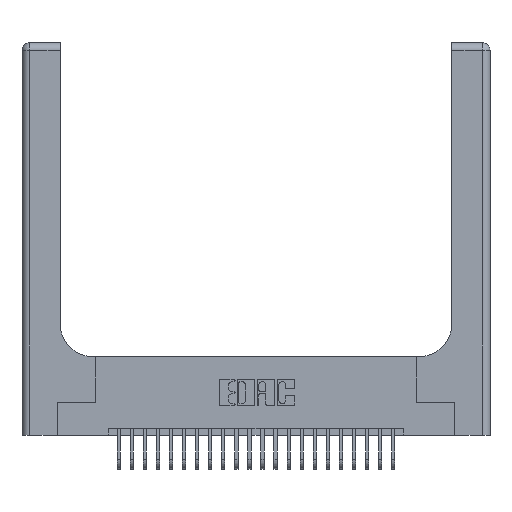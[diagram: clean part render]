
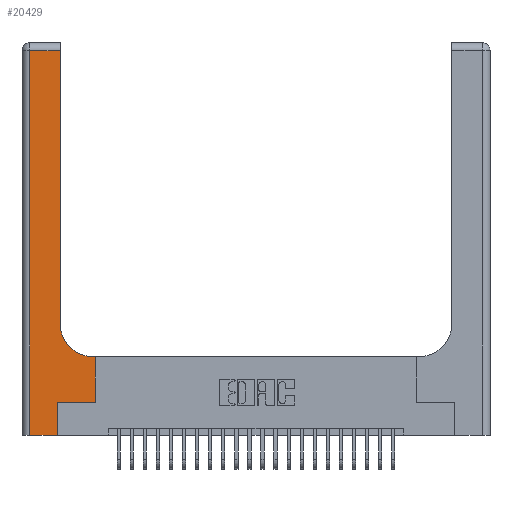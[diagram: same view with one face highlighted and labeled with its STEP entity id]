
A CAD part, top view. The second image highlights one B-rep face of the part: STEP entity #20429.
In plain terms, the highlighted planar face has unit normal (0, 0, 1).
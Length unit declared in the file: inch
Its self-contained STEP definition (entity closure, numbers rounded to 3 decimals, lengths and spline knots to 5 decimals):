
#348 = CARTESIAN_POINT ( 'NONE',  ( 0.2915, 3., 0.37 ) ) ;
#373 = VECTOR ( 'NONE', #18323, 39.37008 ) ;
#494 = ORIENTED_EDGE ( 'NONE', *, *, #7584, .T. ) ;
#872 = CARTESIAN_POINT ( 'NONE',  ( 0.2915, 0.6, 0.37 ) ) ;
#1083 = VECTOR ( 'NONE', #22048, 39.37008 ) ;
#1438 = DIRECTION ( 'NONE',  ( 0., -1., 0. ) ) ;
#1998 = VECTOR ( 'NONE', #5953, 39.37008 ) ;
#2379 = EDGE_CURVE ( 'NONE', #13437, #9790, #12954, .T. ) ;
#2691 = VERTEX_POINT ( 'NONE', #5757 ) ;
#2952 = VECTOR ( 'NONE', #17506, 39.37008 ) ;
#3462 = VECTOR ( 'NONE', #1438, 39.37008 ) ;
#3975 = DIRECTION ( 'NONE',  ( 1., 0., 0. ) ) ;
#4070 = CARTESIAN_POINT ( 'NONE',  ( 0.269, 0.25, 0.37 ) ) ;
#4483 = EDGE_CURVE ( 'NONE', #10352, #2691, #19727, .T. ) ;
#4904 = AXIS2_PLACEMENT_3D ( 'NONE', #17351, #9272, #21619 ) ;
#5395 = CARTESIAN_POINT ( 'NONE',  ( 0.269, 0., 0.37 ) ) ;
#5524 = FACE_OUTER_BOUND ( 'NONE', #23906, .T. ) ;
#5757 = CARTESIAN_POINT ( 'NONE',  ( 0.2915, 2.94, 0.37 ) ) ;
#5821 = DIRECTION ( 'NONE',  ( 1., 0., 0. ) ) ;
#5953 = DIRECTION ( 'NONE',  ( -1., 0., 0. ) ) ;
#6017 = LINE ( 'NONE', #18835, #8884 ) ;
#6260 = ORIENTED_EDGE ( 'NONE', *, *, #2379, .T. ) ;
#6697 = DIRECTION ( 'NONE',  ( 0., 1., 0. ) ) ;
#6886 = VERTEX_POINT ( 'NONE', #24408 ) ;
#7006 = CARTESIAN_POINT ( 'NONE',  ( 0.5585, 0.25, 0.37 ) ) ;
#7324 = CARTESIAN_POINT ( 'NONE',  ( 0.5585, 0.6, 0.37 ) ) ;
#7468 = VERTEX_POINT ( 'NONE', #17929 ) ;
#7551 = CARTESIAN_POINT ( 'NONE',  ( 0.5415, 0.6, 0.37 ) ) ;
#7584 = EDGE_CURVE ( 'NONE', #19217, #7468, #12005, .T. ) ;
#7746 = ORIENTED_EDGE ( 'NONE', *, *, #4483, .T. ) ;
#8631 = ORIENTED_EDGE ( 'NONE', *, *, #8891, .T. ) ;
#8880 = CARTESIAN_POINT ( 'NONE',  ( 0., 0., 0.37 ) ) ;
#8884 = VECTOR ( 'NONE', #6697, 39.37008 ) ;
#8891 = EDGE_CURVE ( 'NONE', #16024, #10560, #21038, .T. ) ;
#9272 = DIRECTION ( 'NONE',  ( 0., 0., -1. ) ) ;
#9406 = LINE ( 'NONE', #16996, #1998 ) ;
#9558 = LINE ( 'NONE', #24699, #3462 ) ;
#9790 = VERTEX_POINT ( 'NONE', #7551 ) ;
#9895 = ORIENTED_EDGE ( 'NONE', *, *, #23053, .T. ) ;
#10352 = VERTEX_POINT ( 'NONE', #20778 ) ;
#10560 = VERTEX_POINT ( 'NONE', #7006 ) ;
#10814 = EDGE_CURVE ( 'NONE', #6886, #19217, #9558, .T. ) ;
#10917 = VECTOR ( 'NONE', #14787, 39.37008 ) ;
#12005 = LINE ( 'NONE', #8880, #373 ) ;
#12451 = ORIENTED_EDGE ( 'NONE', *, *, #15175, .T. ) ;
#12764 = CIRCLE ( 'NONE', #25230, 0.25 ) ;
#12954 = LINE ( 'NONE', #872, #2952 ) ;
#13437 = VERTEX_POINT ( 'NONE', #7324 ) ;
#14045 = DIRECTION ( 'NONE',  ( 0., 0., -1. ) ) ;
#14787 = DIRECTION ( 'NONE',  ( 0., 1., 0. ) ) ;
#15175 = EDGE_CURVE ( 'NONE', #2691, #6886, #9406, .T. ) ;
#15218 = CARTESIAN_POINT ( 'NONE',  ( 0.269, 0.25, 0.37 ) ) ;
#16024 = VERTEX_POINT ( 'NONE', #15218 ) ;
#16996 = CARTESIAN_POINT ( 'NONE',  ( 0., 2.94, 0.37 ) ) ;
#17351 = CARTESIAN_POINT ( 'NONE',  ( 0., 3., 0.37 ) ) ;
#17506 = DIRECTION ( 'NONE',  ( -1., 0., 0. ) ) ;
#17929 = CARTESIAN_POINT ( 'NONE',  ( 0.269, 0., 0.37 ) ) ;
#18323 = DIRECTION ( 'NONE',  ( 1., 0., 0. ) ) ;
#18835 = CARTESIAN_POINT ( 'NONE',  ( 0.5585, 0.25, 0.37 ) ) ;
#19040 = EDGE_CURVE ( 'NONE', #10560, #13437, #6017, .T. ) ;
#19217 = VERTEX_POINT ( 'NONE', #19373 ) ;
#19373 = CARTESIAN_POINT ( 'NONE',  ( 0.06, 0., 0.37 ) ) ;
#19727 = LINE ( 'NONE', #348, #10917 ) ;
#20429 = ADVANCED_FACE ( 'NONE', ( #5524 ), #21436, .F. ) ;
#20661 = ORIENTED_EDGE ( 'NONE', *, *, #19040, .T. ) ;
#20778 = CARTESIAN_POINT ( 'NONE',  ( 0.2915, 0.85, 0.37 ) ) ;
#21038 = LINE ( 'NONE', #4070, #25264 ) ;
#21122 = EDGE_CURVE ( 'NONE', #9790, #10352, #12764, .T. ) ;
#21436 = PLANE ( 'NONE',  #4904 ) ;
#21619 = DIRECTION ( 'NONE',  ( -1., 0., 0. ) ) ;
#22034 = CARTESIAN_POINT ( 'NONE',  ( 0.5415, 0.85, 0.37 ) ) ;
#22048 = DIRECTION ( 'NONE',  ( 0., 1., 0. ) ) ;
#22309 = ORIENTED_EDGE ( 'NONE', *, *, #21122, .T. ) ;
#23053 = EDGE_CURVE ( 'NONE', #7468, #16024, #26024, .T. ) ;
#23906 = EDGE_LOOP ( 'NONE', ( #7746, #12451, #25083, #494, #9895, #8631, #20661, #6260, #22309 ) ) ;
#24408 = CARTESIAN_POINT ( 'NONE',  ( 0.06, 2.94, 0.37 ) ) ;
#24699 = CARTESIAN_POINT ( 'NONE',  ( 0.06, 3., 0.37 ) ) ;
#25083 = ORIENTED_EDGE ( 'NONE', *, *, #10814, .T. ) ;
#25230 = AXIS2_PLACEMENT_3D ( 'NONE', #22034, #14045, #5821 ) ;
#25264 = VECTOR ( 'NONE', #3975, 39.37008 ) ;
#26024 = LINE ( 'NONE', #5395, #1083 ) ;
